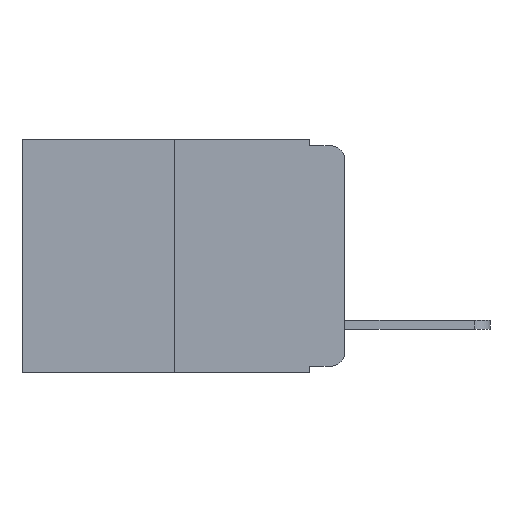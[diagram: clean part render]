
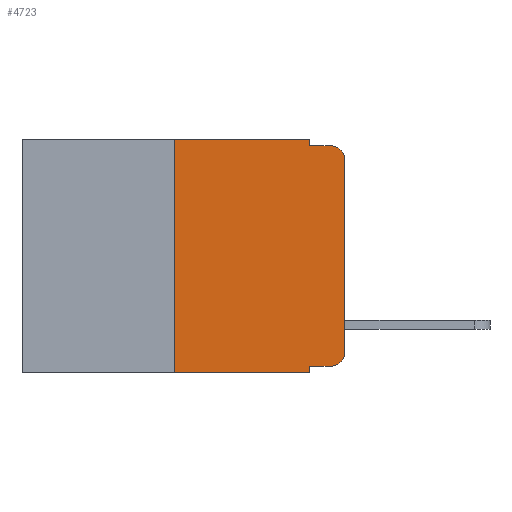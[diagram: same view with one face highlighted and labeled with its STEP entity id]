
A CAD part, left-side view. The second image highlights one B-rep face of the part: STEP entity #4723.
In plain terms, the highlighted planar face has unit normal (-1, 0, 0).
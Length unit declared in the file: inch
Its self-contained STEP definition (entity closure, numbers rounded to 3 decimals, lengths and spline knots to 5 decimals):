
#367 = EDGE_CURVE ( 'NONE', #8576, #6138, #12196, .T. ) ;
#433 = VERTEX_POINT ( 'NONE', #6877 ) ;
#465 = VECTOR ( 'NONE', #5460, 39.37008 ) ;
#509 = EDGE_CURVE ( 'NONE', #10866, #2885, #5701, .T. ) ;
#976 = CARTESIAN_POINT ( 'NONE',  ( 0., 0.25, 0. ) ) ;
#1269 = VERTEX_POINT ( 'NONE', #3191 ) ;
#1349 = EDGE_LOOP ( 'NONE', ( #8174, #8288, #8427, #8603, #8748, #8761, #10592, #6267, #10107, #9701 ) ) ;
#1577 = LINE ( 'NONE', #7095, #8659 ) ;
#2057 = CARTESIAN_POINT ( 'NONE',  ( 0., 0.051, -0.01 ) ) ;
#2158 = VECTOR ( 'NONE', #6574, 39.37008 ) ;
#2241 = CARTESIAN_POINT ( 'NONE',  ( 0., 0.02, -0.313 ) ) ;
#2633 = EDGE_CURVE ( 'NONE', #433, #9942, #10700, .T. ) ;
#2709 = CARTESIAN_POINT ( 'NONE',  ( 0., 0.051, 0. ) ) ;
#2838 = FACE_OUTER_BOUND ( 'NONE', #1349, .T. ) ;
#2885 = VERTEX_POINT ( 'NONE', #12268 ) ;
#3103 = DIRECTION ( 'NONE',  ( -1., 0., 0. ) ) ;
#3191 = CARTESIAN_POINT ( 'NONE',  ( 0., 0.02, -0.01 ) ) ;
#3302 = VECTOR ( 'NONE', #9211, 39.37008 ) ;
#3370 = CARTESIAN_POINT ( 'NONE',  ( 0., 0., -0.03 ) ) ;
#3399 = CARTESIAN_POINT ( 'NONE',  ( 0., 0.051, 0. ) ) ;
#3589 = DIRECTION ( 'NONE',  ( 0., 0., -1. ) ) ;
#4184 = CARTESIAN_POINT ( 'NONE',  ( 0., 0.02, -0.03 ) ) ;
#4244 = CARTESIAN_POINT ( 'NONE',  ( 0., 0.051, -0.333 ) ) ;
#4408 = LINE ( 'NONE', #2057, #11117 ) ;
#4578 = VERTEX_POINT ( 'NONE', #10095 ) ;
#4620 = AXIS2_PLACEMENT_3D ( 'NONE', #5681, #11074, #6367 ) ;
#4723 = ADVANCED_FACE ( 'NONE', ( #2838 ), #6545, .F. ) ;
#4800 = DIRECTION ( 'NONE',  ( 0., -1., 0. ) ) ;
#5221 = DIRECTION ( 'NONE',  ( 0., 0., -1. ) ) ;
#5222 = DIRECTION ( 'NONE',  ( 0., -1., 0. ) ) ;
#5460 = DIRECTION ( 'NONE',  ( 0., 0., 1. ) ) ;
#5603 = CARTESIAN_POINT ( 'NONE',  ( 0., 0.473, -0.343 ) ) ;
#5681 = CARTESIAN_POINT ( 'NONE',  ( 0., 0.473, 0. ) ) ;
#5701 = LINE ( 'NONE', #2709, #7979 ) ;
#5756 = CIRCLE ( 'NONE', #5837, 0.02 ) ;
#5837 = AXIS2_PLACEMENT_3D ( 'NONE', #4184, #10658, #5221 ) ;
#5943 = VECTOR ( 'NONE', #4800, 39.37008 ) ;
#6138 = VERTEX_POINT ( 'NONE', #3370 ) ;
#6146 = LINE ( 'NONE', #976, #465 ) ;
#6208 = CARTESIAN_POINT ( 'NONE',  ( 0., 0.02, -0.333 ) ) ;
#6267 = ORIENTED_EDGE ( 'NONE', *, *, #509, .F. ) ;
#6268 = EDGE_CURVE ( 'NONE', #10866, #10798, #1577, .T. ) ;
#6367 = DIRECTION ( 'NONE',  ( 0., 0., -1. ) ) ;
#6545 = PLANE ( 'NONE',  #4620 ) ;
#6574 = DIRECTION ( 'NONE',  ( 0., -1., 0. ) ) ;
#6604 = EDGE_CURVE ( 'NONE', #10798, #8576, #7043, .T. ) ;
#6877 = CARTESIAN_POINT ( 'NONE',  ( 0., 0.25, 0. ) ) ;
#7043 = CIRCLE ( 'NONE', #7122, 0.02 ) ;
#7095 = CARTESIAN_POINT ( 'NONE',  ( 0., 0.051, -0.333 ) ) ;
#7101 = DIRECTION ( 'NONE',  ( 0., -1., 0. ) ) ;
#7122 = AXIS2_PLACEMENT_3D ( 'NONE', #2241, #3103, #3589 ) ;
#7213 = VECTOR ( 'NONE', #11162, 39.37008 ) ;
#7715 = EDGE_CURVE ( 'NONE', #6138, #1269, #5756, .T. ) ;
#7979 = VECTOR ( 'NONE', #10547, 39.37008 ) ;
#8174 = ORIENTED_EDGE ( 'NONE', *, *, #367, .T. ) ;
#8288 = ORIENTED_EDGE ( 'NONE', *, *, #7715, .T. ) ;
#8402 = CARTESIAN_POINT ( 'NONE',  ( 0., 0.051, -0.01 ) ) ;
#8427 = ORIENTED_EDGE ( 'NONE', *, *, #10667, .F. ) ;
#8573 = VERTEX_POINT ( 'NONE', #8402 ) ;
#8576 = VERTEX_POINT ( 'NONE', #10070 ) ;
#8603 = ORIENTED_EDGE ( 'NONE', *, *, #11041, .F. ) ;
#8659 = VECTOR ( 'NONE', #7101, 39.37008 ) ;
#8663 = EDGE_CURVE ( 'NONE', #4578, #2885, #11020, .T. ) ;
#8748 = ORIENTED_EDGE ( 'NONE', *, *, #2633, .F. ) ;
#8761 = ORIENTED_EDGE ( 'NONE', *, *, #12289, .F. ) ;
#9211 = DIRECTION ( 'NONE',  ( 0., 0., -1. ) ) ;
#9413 = CARTESIAN_POINT ( 'NONE',  ( 0., 0.051, 0. ) ) ;
#9701 = ORIENTED_EDGE ( 'NONE', *, *, #6604, .T. ) ;
#9942 = VERTEX_POINT ( 'NONE', #9413 ) ;
#10070 = CARTESIAN_POINT ( 'NONE',  ( 0., 0., -0.313 ) ) ;
#10095 = CARTESIAN_POINT ( 'NONE',  ( 0., 0.25, -0.343 ) ) ;
#10107 = ORIENTED_EDGE ( 'NONE', *, *, #6268, .T. ) ;
#10484 = LINE ( 'NONE', #3399, #3302 ) ;
#10547 = DIRECTION ( 'NONE',  ( 0., 0., -1. ) ) ;
#10592 = ORIENTED_EDGE ( 'NONE', *, *, #8663, .T. ) ;
#10605 = CARTESIAN_POINT ( 'NONE',  ( 0., 0.473, 0. ) ) ;
#10658 = DIRECTION ( 'NONE',  ( -1., 0., 0. ) ) ;
#10667 = EDGE_CURVE ( 'NONE', #8573, #1269, #4408, .T. ) ;
#10700 = LINE ( 'NONE', #10605, #5943 ) ;
#10798 = VERTEX_POINT ( 'NONE', #6208 ) ;
#10866 = VERTEX_POINT ( 'NONE', #4244 ) ;
#11020 = LINE ( 'NONE', #5603, #2158 ) ;
#11041 = EDGE_CURVE ( 'NONE', #9942, #8573, #10484, .T. ) ;
#11074 = DIRECTION ( 'NONE',  ( 1., 0., 0. ) ) ;
#11117 = VECTOR ( 'NONE', #5222, 39.37008 ) ;
#11144 = CARTESIAN_POINT ( 'NONE',  ( 0., 0., 0. ) ) ;
#11162 = DIRECTION ( 'NONE',  ( 0., 0., 1. ) ) ;
#12196 = LINE ( 'NONE', #11144, #7213 ) ;
#12268 = CARTESIAN_POINT ( 'NONE',  ( 0., 0.051, -0.343 ) ) ;
#12289 = EDGE_CURVE ( 'NONE', #4578, #433, #6146, .T. ) ;
